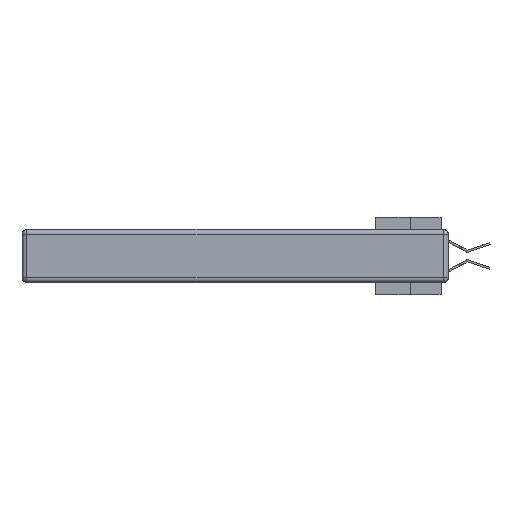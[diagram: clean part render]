
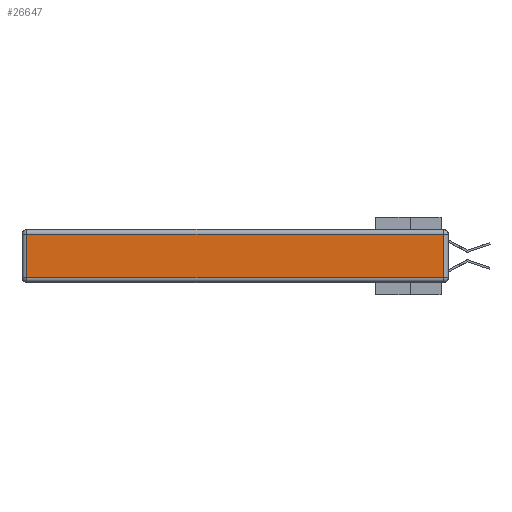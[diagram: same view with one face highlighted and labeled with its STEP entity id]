
A CAD part, left-side view. The second image highlights one B-rep face of the part: STEP entity #26647.
In plain terms, the highlighted planar face has unit normal (-1, 0, 0).
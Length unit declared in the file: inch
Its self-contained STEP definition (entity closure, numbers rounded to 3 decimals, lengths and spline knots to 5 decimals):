
#1744 = EDGE_CURVE ( 'NONE', #19513, #11710, #29605, .T. ) ;
#2495 = CARTESIAN_POINT ( 'NONE',  ( 0., 2.72, -0.313 ) ) ;
#5894 = DIRECTION ( 'NONE',  ( 0., 0., 1. ) ) ;
#5924 = ORIENTED_EDGE ( 'NONE', *, *, #1744, .T. ) ;
#6701 = AXIS2_PLACEMENT_3D ( 'NONE', #26516, #29703, #5894 ) ;
#8348 = VECTOR ( 'NONE', #17744, 39.37008 ) ;
#8959 = PLANE ( 'NONE',  #6701 ) ;
#10685 = DIRECTION ( 'NONE',  ( 0., 0., 1. ) ) ;
#10882 = CARTESIAN_POINT ( 'NONE',  ( 0., 2.75, -0.03 ) ) ;
#11495 = EDGE_CURVE ( 'NONE', #28036, #15810, #17626, .T. ) ;
#11710 = VERTEX_POINT ( 'NONE', #2495 ) ;
#12788 = CARTESIAN_POINT ( 'NONE',  ( 0., 0.03, -0.03 ) ) ;
#15810 = VERTEX_POINT ( 'NONE', #12788 ) ;
#16487 = EDGE_CURVE ( 'NONE', #15810, #19513, #20279, .T. ) ;
#16600 = FACE_OUTER_BOUND ( 'NONE', #31372, .T. ) ;
#17626 = LINE ( 'NONE', #28443, #26875 ) ;
#17744 = DIRECTION ( 'NONE',  ( 0., -1., 0. ) ) ;
#17868 = ORIENTED_EDGE ( 'NONE', *, *, #11495, .T. ) ;
#18539 = VECTOR ( 'NONE', #27521, 39.37008 ) ;
#18683 = ORIENTED_EDGE ( 'NONE', *, *, #16487, .T. ) ;
#19513 = VERTEX_POINT ( 'NONE', #35999 ) ;
#20279 = LINE ( 'NONE', #10882, #33157 ) ;
#23569 = EDGE_CURVE ( 'NONE', #11710, #28036, #34802, .T. ) ;
#23956 = CARTESIAN_POINT ( 'NONE',  ( 0., 0., -0.313 ) ) ;
#25817 = DIRECTION ( 'NONE',  ( 0., 1., 0. ) ) ;
#26516 = CARTESIAN_POINT ( 'NONE',  ( 0., 0., -0.343 ) ) ;
#26647 = ADVANCED_FACE ( 'NONE', ( #16600 ), #8959, .T. ) ;
#26875 = VECTOR ( 'NONE', #10685, 39.37008 ) ;
#27521 = DIRECTION ( 'NONE',  ( 0., 0., -1. ) ) ;
#28036 = VERTEX_POINT ( 'NONE', #35716 ) ;
#28443 = CARTESIAN_POINT ( 'NONE',  ( 0., 0.03, -0.343 ) ) ;
#29605 = LINE ( 'NONE', #33101, #18539 ) ;
#29703 = DIRECTION ( 'NONE',  ( -1., 0., 0. ) ) ;
#31372 = EDGE_LOOP ( 'NONE', ( #34120, #17868, #18683, #5924 ) ) ;
#33101 = CARTESIAN_POINT ( 'NONE',  ( 0., 2.72, -0.343 ) ) ;
#33157 = VECTOR ( 'NONE', #25817, 39.37008 ) ;
#34120 = ORIENTED_EDGE ( 'NONE', *, *, #23569, .T. ) ;
#34802 = LINE ( 'NONE', #23956, #8348 ) ;
#35716 = CARTESIAN_POINT ( 'NONE',  ( 0., 0.03, -0.313 ) ) ;
#35999 = CARTESIAN_POINT ( 'NONE',  ( 0., 2.72, -0.03 ) ) ;
